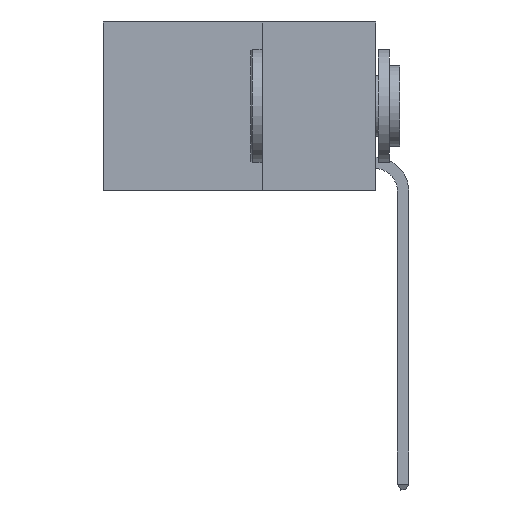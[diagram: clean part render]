
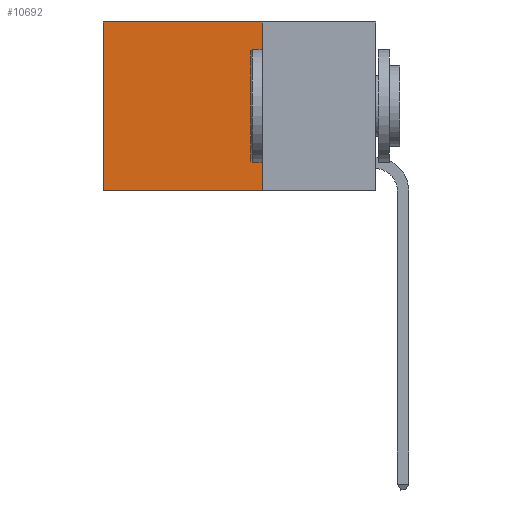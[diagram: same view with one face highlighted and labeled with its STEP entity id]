
A CAD part, left-side view. The second image highlights one B-rep face of the part: STEP entity #10692.
In plain terms, the highlighted planar face has unit normal (-1, 0, 0).
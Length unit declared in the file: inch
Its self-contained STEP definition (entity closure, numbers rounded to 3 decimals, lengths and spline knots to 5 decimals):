
#958 = PLANE ( 'NONE',  #4637 ) ;
#1129 = ORIENTED_EDGE ( 'NONE', *, *, #6129, .T. ) ;
#2200 = DIRECTION ( 'NONE',  ( 0., 0., -1. ) ) ;
#2466 = CARTESIAN_POINT ( 'NONE',  ( 0.2625, 0.25, 0. ) ) ;
#2555 = CARTESIAN_POINT ( 'NONE',  ( 0.2625, 0.6, 0. ) ) ;
#3382 = VECTOR ( 'NONE', #3638, 39.37008 ) ;
#3638 = DIRECTION ( 'NONE',  ( 0., 1., 0. ) ) ;
#3709 = CARTESIAN_POINT ( 'NONE',  ( 0.2625, 0.25, 0. ) ) ;
#3717 = EDGE_CURVE ( 'NONE', #14530, #5945, #13909, .T. ) ;
#4032 = CARTESIAN_POINT ( 'NONE',  ( 0.2625, 0.25, 0. ) ) ;
#4479 = LINE ( 'NONE', #6249, #13300 ) ;
#4637 = AXIS2_PLACEMENT_3D ( 'NONE', #11509, #9261, #2200 ) ;
#4932 = CARTESIAN_POINT ( 'NONE',  ( 0.2625, 0.6, -0.37 ) ) ;
#5232 = DIRECTION ( 'NONE',  ( 0., 0., -1. ) ) ;
#5626 = FACE_OUTER_BOUND ( 'NONE', #10480, .T. ) ;
#5945 = VERTEX_POINT ( 'NONE', #4932 ) ;
#6098 = ORIENTED_EDGE ( 'NONE', *, *, #3717, .F. ) ;
#6129 = EDGE_CURVE ( 'NONE', #6594, #9156, #12639, .T. ) ;
#6192 = CARTESIAN_POINT ( 'NONE',  ( 0.2625, 0.25, -0.37 ) ) ;
#6249 = CARTESIAN_POINT ( 'NONE',  ( 0.2625, 0.6, 0. ) ) ;
#6594 = VERTEX_POINT ( 'NONE', #2466 ) ;
#7424 = DIRECTION ( 'NONE',  ( 0., 0., -1. ) ) ;
#8840 = LINE ( 'NONE', #4032, #11153 ) ;
#9156 = VERTEX_POINT ( 'NONE', #2555 ) ;
#9261 = DIRECTION ( 'NONE',  ( 1., 0., 0. ) ) ;
#10480 = EDGE_LOOP ( 'NONE', ( #11450, #6098, #12076, #1129 ) ) ;
#10692 = ADVANCED_FACE ( 'NONE', ( #5626 ), #958, .F. ) ;
#11153 = VECTOR ( 'NONE', #5232, 39.37008 ) ;
#11450 = ORIENTED_EDGE ( 'NONE', *, *, #12112, .T. ) ;
#11509 = CARTESIAN_POINT ( 'NONE',  ( 0.2625, 0.25, 0. ) ) ;
#12076 = ORIENTED_EDGE ( 'NONE', *, *, #12740, .F. ) ;
#12112 = EDGE_CURVE ( 'NONE', #9156, #5945, #4479, .T. ) ;
#12639 = LINE ( 'NONE', #3709, #3382 ) ;
#12740 = EDGE_CURVE ( 'NONE', #6594, #14530, #8840, .T. ) ;
#13300 = VECTOR ( 'NONE', #7424, 39.37008 ) ;
#13428 = CARTESIAN_POINT ( 'NONE',  ( 0.2625, 0.25, -0.37 ) ) ;
#13516 = DIRECTION ( 'NONE',  ( 0., 1., 0. ) ) ;
#13909 = LINE ( 'NONE', #13428, #14270 ) ;
#14270 = VECTOR ( 'NONE', #13516, 39.37008 ) ;
#14530 = VERTEX_POINT ( 'NONE', #6192 ) ;
